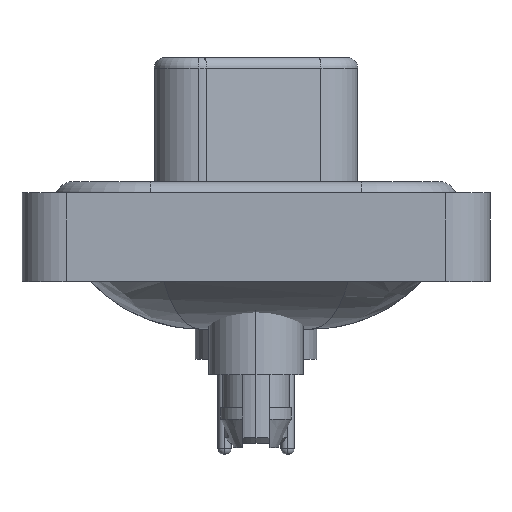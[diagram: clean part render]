
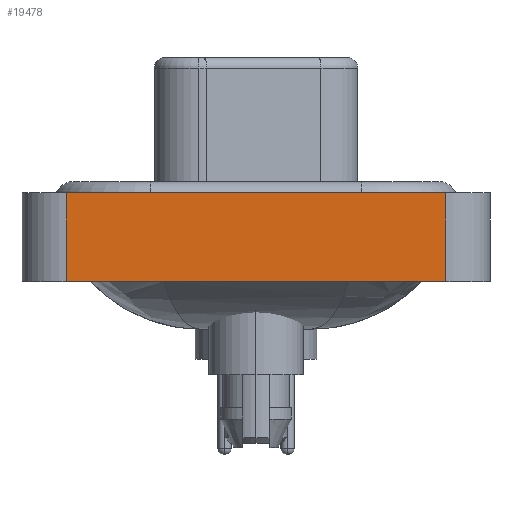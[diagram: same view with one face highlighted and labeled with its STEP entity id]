
A CAD part, left-side view. The second image highlights one B-rep face of the part: STEP entity #19478.
In plain terms, the highlighted planar face has unit normal (-1, 0, 0).
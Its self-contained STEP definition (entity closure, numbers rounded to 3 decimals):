
#51 = EDGE_CURVE ( 'NONE', #13498, #10258, #5214, .T. ) ;
#79 = CARTESIAN_POINT ( 'NONE',  ( -7.35, -8.55, -3.6 ) ) ;
#299 = DIRECTION ( 'NONE',  ( 0., -1., 0. ) ) ;
#3601 = CARTESIAN_POINT ( 'NONE',  ( -7.35, 8.55, -3.6 ) ) ;
#3800 = CARTESIAN_POINT ( 'NONE',  ( -7.35, -8.55, 0.4 ) ) ;
#4792 = CARTESIAN_POINT ( 'NONE',  ( -7.35, 8.55, -3.6 ) ) ;
#5154 = ORIENTED_EDGE ( 'NONE', *, *, #6720, .T. ) ;
#5214 = LINE ( 'NONE', #20284, #20893 ) ;
#5464 = DIRECTION ( 'NONE',  ( 0., 0., 1. ) ) ;
#6720 = EDGE_CURVE ( 'NONE', #26815, #13498, #10438, .T. ) ;
#7314 = AXIS2_PLACEMENT_3D ( 'NONE', #9618, #11795, #17910 ) ;
#8996 = ORIENTED_EDGE ( 'NONE', *, *, #16521, .F. ) ;
#9618 = CARTESIAN_POINT ( 'NONE',  ( -7.35, -8.55, -3.6 ) ) ;
#10258 = VERTEX_POINT ( 'NONE', #3800 ) ;
#10438 = LINE ( 'NONE', #79, #23953 ) ;
#10784 = ORIENTED_EDGE ( 'NONE', *, *, #51, .T. ) ;
#11795 = DIRECTION ( 'NONE',  ( -1., 0., 0. ) ) ;
#12106 = CARTESIAN_POINT ( 'NONE',  ( -7.35, -8.55, -3.6 ) ) ;
#12568 = CARTESIAN_POINT ( 'NONE',  ( -7.35, -8.55, 0.4 ) ) ;
#13193 = ORIENTED_EDGE ( 'NONE', *, *, #26833, .F. ) ;
#13498 = VERTEX_POINT ( 'NONE', #12106 ) ;
#14071 = VECTOR ( 'NONE', #299, 1000. ) ;
#14223 = FACE_OUTER_BOUND ( 'NONE', #19995, .T. ) ;
#16521 = EDGE_CURVE ( 'NONE', #26815, #22535, #20989, .T. ) ;
#17910 = DIRECTION ( 'NONE',  ( 0., 0., 1. ) ) ;
#18032 = PLANE ( 'NONE',  #7314 ) ;
#19228 = CARTESIAN_POINT ( 'NONE',  ( -7.35, 8.55, 0.4 ) ) ;
#19478 = ADVANCED_FACE ( 'NONE', ( #14223 ), #18032, .T. ) ;
#19562 = VECTOR ( 'NONE', #23286, 1000. ) ;
#19995 = EDGE_LOOP ( 'NONE', ( #10784, #13193, #8996, #5154 ) ) ;
#20284 = CARTESIAN_POINT ( 'NONE',  ( -7.35, -8.55, -3.6 ) ) ;
#20893 = VECTOR ( 'NONE', #5464, 1000. ) ;
#20989 = LINE ( 'NONE', #4792, #19562 ) ;
#21275 = LINE ( 'NONE', #12568, #14071 ) ;
#22535 = VERTEX_POINT ( 'NONE', #19228 ) ;
#23286 = DIRECTION ( 'NONE',  ( 0., 0., 1. ) ) ;
#23953 = VECTOR ( 'NONE', #26880, 1000. ) ;
#26815 = VERTEX_POINT ( 'NONE', #3601 ) ;
#26833 = EDGE_CURVE ( 'NONE', #22535, #10258, #21275, .T. ) ;
#26880 = DIRECTION ( 'NONE',  ( 0., -1., 0. ) ) ;
